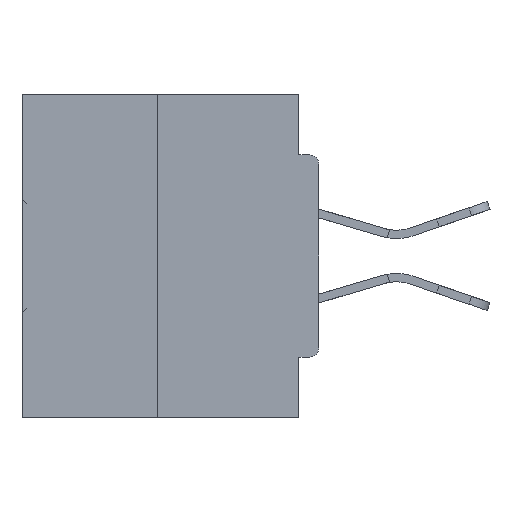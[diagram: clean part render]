
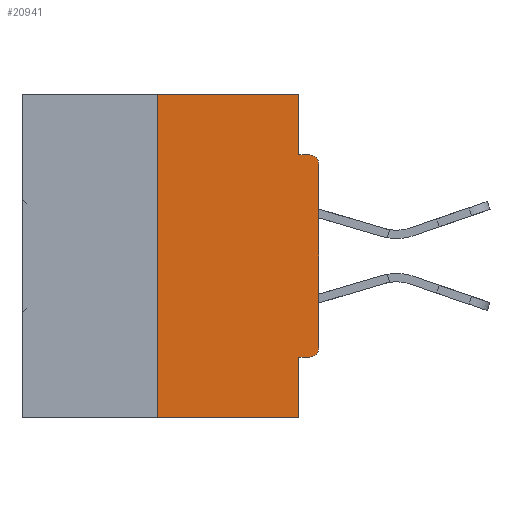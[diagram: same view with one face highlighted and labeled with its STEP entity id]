
A CAD part, left-side view. The second image highlights one B-rep face of the part: STEP entity #20941.
In plain terms, the highlighted planar face has unit normal (-1, 0, 0).
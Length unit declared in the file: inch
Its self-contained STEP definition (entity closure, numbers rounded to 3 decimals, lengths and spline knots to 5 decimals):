
#112 = EDGE_CURVE ( 'NONE', #19466, #27779, #26760, .T. ) ;
#148 = AXIS2_PLACEMENT_3D ( 'NONE', #5150, #26224, #36752 ) ;
#1761 = LINE ( 'NONE', #8330, #19708 ) ;
#1951 = VECTOR ( 'NONE', #11562, 39.37008 ) ;
#2184 = FACE_OUTER_BOUND ( 'NONE', #4817, .T. ) ;
#2206 = VERTEX_POINT ( 'NONE', #39663 ) ;
#2940 = DIRECTION ( 'NONE',  ( 0., 0., 1. ) ) ;
#3006 = LINE ( 'NONE', #8090, #30018 ) ;
#3379 = CARTESIAN_POINT ( 'NONE',  ( 0., 0.25, 0. ) ) ;
#3827 = EDGE_CURVE ( 'NONE', #2206, #23397, #16474, .T. ) ;
#4817 = EDGE_LOOP ( 'NONE', ( #29348, #34930, #27249, #13878, #27602, #26498, #10589, #19992, #23440, #27471 ) ) ;
#5150 = CARTESIAN_POINT ( 'NONE',  ( 0., 0.015, -0.3915 ) ) ;
#5377 = CARTESIAN_POINT ( 'NONE',  ( 0., 0., 0. ) ) ;
#6819 = LINE ( 'NONE', #17893, #28229 ) ;
#7717 = CARTESIAN_POINT ( 'NONE',  ( 0., 0.015, -0.1085 ) ) ;
#8090 = CARTESIAN_POINT ( 'NONE',  ( 0., 0.031, 0. ) ) ;
#8330 = CARTESIAN_POINT ( 'NONE',  ( 0., 0.46, 0. ) ) ;
#9267 = CARTESIAN_POINT ( 'NONE',  ( 0., 0., -0.1085 ) ) ;
#10589 = ORIENTED_EDGE ( 'NONE', *, *, #25647, .T. ) ;
#11411 = DIRECTION ( 'NONE',  ( 0., 0., -1. ) ) ;
#11562 = DIRECTION ( 'NONE',  ( 0., -1., 0. ) ) ;
#11578 = CARTESIAN_POINT ( 'NONE',  ( 0., 0.031, 0. ) ) ;
#11602 = CARTESIAN_POINT ( 'NONE',  ( 0., 0.031, -0.5 ) ) ;
#11698 = VERTEX_POINT ( 'NONE', #17531 ) ;
#11792 = EDGE_CURVE ( 'NONE', #11698, #18556, #1761, .T. ) ;
#12067 = DIRECTION ( 'NONE',  ( 0., 0., -1. ) ) ;
#13878 = ORIENTED_EDGE ( 'NONE', *, *, #112, .F. ) ;
#13921 = VERTEX_POINT ( 'NONE', #42857 ) ;
#15244 = EDGE_CURVE ( 'NONE', #13921, #27779, #26700, .T. ) ;
#15302 = LINE ( 'NONE', #5377, #45124 ) ;
#16200 = DIRECTION ( 'NONE',  ( 0., 0., 1. ) ) ;
#16474 = LINE ( 'NONE', #28512, #22611 ) ;
#17531 = CARTESIAN_POINT ( 'NONE',  ( 0., 0.25, 0. ) ) ;
#17893 = CARTESIAN_POINT ( 'NONE',  ( 0., 0., -0.4065 ) ) ;
#18556 = VERTEX_POINT ( 'NONE', #11578 ) ;
#18586 = CIRCLE ( 'NONE', #24038, 0.015 ) ;
#18682 = DIRECTION ( 'NONE',  ( -1., 0., 0. ) ) ;
#19053 = EDGE_CURVE ( 'NONE', #25013, #23397, #18586, .T. ) ;
#19466 = VERTEX_POINT ( 'NONE', #33810 ) ;
#19708 = VECTOR ( 'NONE', #37299, 39.37008 ) ;
#19992 = ORIENTED_EDGE ( 'NONE', *, *, #19053, .T. ) ;
#20941 = ADVANCED_FACE ( 'NONE', ( #2184 ), #42618, .F. ) ;
#21087 = DIRECTION ( 'NONE',  ( 0., 0., -1. ) ) ;
#21372 = DIRECTION ( 'NONE',  ( 0., -1., 0. ) ) ;
#22245 = CARTESIAN_POINT ( 'NONE',  ( 0., 0.46, -0.5 ) ) ;
#22611 = VECTOR ( 'NONE', #21372, 39.37008 ) ;
#23397 = VERTEX_POINT ( 'NONE', #32520 ) ;
#23440 = ORIENTED_EDGE ( 'NONE', *, *, #3827, .F. ) ;
#24038 = AXIS2_PLACEMENT_3D ( 'NONE', #7717, #18682, #32889 ) ;
#25013 = VERTEX_POINT ( 'NONE', #9267 ) ;
#25647 = EDGE_CURVE ( 'NONE', #42882, #25013, #15302, .T. ) ;
#25666 = VECTOR ( 'NONE', #2940, 39.37008 ) ;
#26224 = DIRECTION ( 'NONE',  ( -1., 0., 0. ) ) ;
#26498 = ORIENTED_EDGE ( 'NONE', *, *, #28022, .T. ) ;
#26700 = LINE ( 'NONE', #22245, #1951 ) ;
#26760 = LINE ( 'NONE', #11602, #38558 ) ;
#27249 = ORIENTED_EDGE ( 'NONE', *, *, #15244, .T. ) ;
#27471 = ORIENTED_EDGE ( 'NONE', *, *, #42665, .F. ) ;
#27602 = ORIENTED_EDGE ( 'NONE', *, *, #43613, .F. ) ;
#27774 = CARTESIAN_POINT ( 'NONE',  ( 0., 0.031, -0.5 ) ) ;
#27779 = VERTEX_POINT ( 'NONE', #27774 ) ;
#28022 = EDGE_CURVE ( 'NONE', #32558, #42882, #32651, .T. ) ;
#28229 = VECTOR ( 'NONE', #28655, 39.37008 ) ;
#28512 = CARTESIAN_POINT ( 'NONE',  ( 0., 0., -0.0935 ) ) ;
#28655 = DIRECTION ( 'NONE',  ( 0., 1., 0. ) ) ;
#29348 = ORIENTED_EDGE ( 'NONE', *, *, #11792, .F. ) ;
#30018 = VECTOR ( 'NONE', #11411, 39.37008 ) ;
#30794 = LINE ( 'NONE', #3379, #25666 ) ;
#32520 = CARTESIAN_POINT ( 'NONE',  ( 0., 0.015, -0.0935 ) ) ;
#32558 = VERTEX_POINT ( 'NONE', #39849 ) ;
#32651 = CIRCLE ( 'NONE', #148, 0.015 ) ;
#32889 = DIRECTION ( 'NONE',  ( 0., 0., -1. ) ) ;
#33073 = CARTESIAN_POINT ( 'NONE',  ( 0., 0., -0.3915 ) ) ;
#33810 = CARTESIAN_POINT ( 'NONE',  ( 0., 0.031, -0.4065 ) ) ;
#34930 = ORIENTED_EDGE ( 'NONE', *, *, #40942, .F. ) ;
#35450 = DIRECTION ( 'NONE',  ( 1., 0., 0. ) ) ;
#36752 = DIRECTION ( 'NONE',  ( 0., 0., -1. ) ) ;
#37299 = DIRECTION ( 'NONE',  ( 0., -1., 0. ) ) ;
#38558 = VECTOR ( 'NONE', #12067, 39.37008 ) ;
#39663 = CARTESIAN_POINT ( 'NONE',  ( 0., 0.031, -0.0935 ) ) ;
#39849 = CARTESIAN_POINT ( 'NONE',  ( 0., 0.015, -0.4065 ) ) ;
#40916 = AXIS2_PLACEMENT_3D ( 'NONE', #45779, #35450, #21087 ) ;
#40942 = EDGE_CURVE ( 'NONE', #13921, #11698, #30794, .T. ) ;
#42618 = PLANE ( 'NONE',  #40916 ) ;
#42665 = EDGE_CURVE ( 'NONE', #18556, #2206, #3006, .T. ) ;
#42857 = CARTESIAN_POINT ( 'NONE',  ( 0., 0.25, -0.5 ) ) ;
#42882 = VERTEX_POINT ( 'NONE', #33073 ) ;
#43613 = EDGE_CURVE ( 'NONE', #32558, #19466, #6819, .T. ) ;
#45124 = VECTOR ( 'NONE', #16200, 39.37008 ) ;
#45779 = CARTESIAN_POINT ( 'NONE',  ( 0., 0.46, 0. ) ) ;
